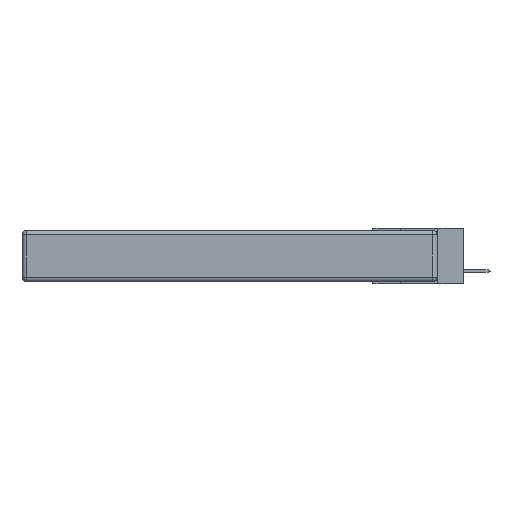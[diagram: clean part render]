
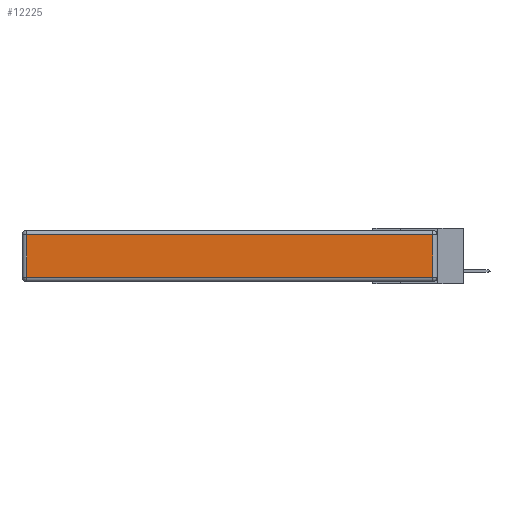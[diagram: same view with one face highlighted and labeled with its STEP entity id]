
A CAD part, left-side view. The second image highlights one B-rep face of the part: STEP entity #12225.
In plain terms, the highlighted planar face has unit normal (-1, 0, 0).
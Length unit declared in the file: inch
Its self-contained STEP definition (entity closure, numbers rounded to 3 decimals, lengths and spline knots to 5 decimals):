
#144 = VERTEX_POINT ( 'NONE', #17266 ) ;
#454 = ORIENTED_EDGE ( 'NONE', *, *, #11113, .T. ) ;
#1131 = CARTESIAN_POINT ( 'NONE',  ( 0., 2.72, -0.343 ) ) ;
#1825 = CARTESIAN_POINT ( 'NONE',  ( 0., 0., -0.343 ) ) ;
#2199 = DIRECTION ( 'NONE',  ( 0., 0., 1. ) ) ;
#2625 = CARTESIAN_POINT ( 'NONE',  ( 0., 2.72, -0.03 ) ) ;
#3229 = DIRECTION ( 'NONE',  ( 0., 0., 1. ) ) ;
#4362 = LINE ( 'NONE', #5093, #17305 ) ;
#4449 = DIRECTION ( 'NONE',  ( -1., 0., 0. ) ) ;
#4556 = DIRECTION ( 'NONE',  ( 0., 1., 0. ) ) ;
#4633 = PLANE ( 'NONE',  #7792 ) ;
#4660 = LINE ( 'NONE', #7080, #15391 ) ;
#5093 = CARTESIAN_POINT ( 'NONE',  ( 0., 0.03, -0.343 ) ) ;
#5498 = DIRECTION ( 'NONE',  ( 0., 0., -1. ) ) ;
#5553 = LINE ( 'NONE', #12836, #12575 ) ;
#6919 = VERTEX_POINT ( 'NONE', #17031 ) ;
#7080 = CARTESIAN_POINT ( 'NONE',  ( 0., 2.75, -0.03 ) ) ;
#7769 = VERTEX_POINT ( 'NONE', #2625 ) ;
#7792 = AXIS2_PLACEMENT_3D ( 'NONE', #1825, #4449, #3229 ) ;
#8557 = EDGE_CURVE ( 'NONE', #6919, #7769, #4660, .T. ) ;
#8747 = LINE ( 'NONE', #1131, #14417 ) ;
#10210 = EDGE_CURVE ( 'NONE', #16133, #6919, #4362, .T. ) ;
#11113 = EDGE_CURVE ( 'NONE', #7769, #144, #8747, .T. ) ;
#11142 = ORIENTED_EDGE ( 'NONE', *, *, #10210, .T. ) ;
#12160 = ORIENTED_EDGE ( 'NONE', *, *, #8557, .T. ) ;
#12212 = FACE_OUTER_BOUND ( 'NONE', #12433, .T. ) ;
#12225 = ADVANCED_FACE ( 'NONE', ( #12212 ), #4633, .T. ) ;
#12433 = EDGE_LOOP ( 'NONE', ( #16304, #11142, #12160, #454 ) ) ;
#12575 = VECTOR ( 'NONE', #12780, 39.37008 ) ;
#12780 = DIRECTION ( 'NONE',  ( 0., -1., 0. ) ) ;
#12836 = CARTESIAN_POINT ( 'NONE',  ( 0., 0., -0.313 ) ) ;
#14417 = VECTOR ( 'NONE', #5498, 39.37008 ) ;
#14758 = EDGE_CURVE ( 'NONE', #144, #16133, #5553, .T. ) ;
#15153 = CARTESIAN_POINT ( 'NONE',  ( 0., 0.03, -0.313 ) ) ;
#15391 = VECTOR ( 'NONE', #4556, 39.37008 ) ;
#16133 = VERTEX_POINT ( 'NONE', #15153 ) ;
#16304 = ORIENTED_EDGE ( 'NONE', *, *, #14758, .T. ) ;
#17031 = CARTESIAN_POINT ( 'NONE',  ( 0., 0.03, -0.03 ) ) ;
#17266 = CARTESIAN_POINT ( 'NONE',  ( 0., 2.72, -0.313 ) ) ;
#17305 = VECTOR ( 'NONE', #2199, 39.37008 ) ;
